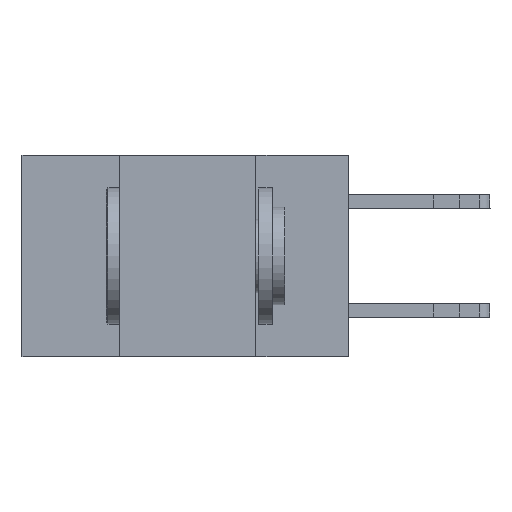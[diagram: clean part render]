
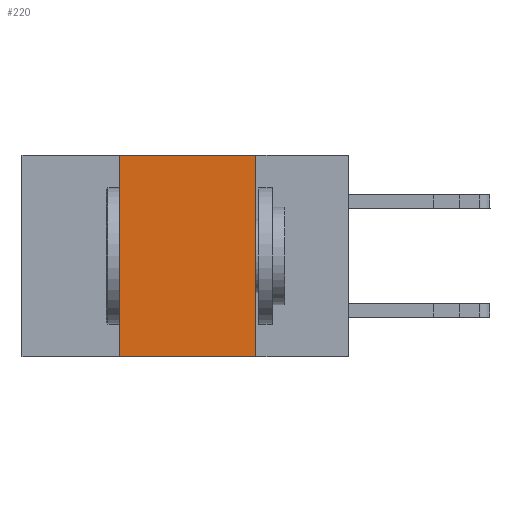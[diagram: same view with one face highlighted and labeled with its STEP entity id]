
A CAD part, left-side view. The second image highlights one B-rep face of the part: STEP entity #220.
In plain terms, the highlighted planar face has unit normal (-1, 0, 0).
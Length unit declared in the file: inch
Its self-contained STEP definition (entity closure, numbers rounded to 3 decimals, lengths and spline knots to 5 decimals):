
#20 = VECTOR ( 'NONE', #7049, 39.37008 ) ;
#220 = ADVANCED_FACE ( 'NONE', ( #6850 ), #9787, .F. ) ;
#585 = CARTESIAN_POINT ( 'NONE',  ( 0., 0.17, 0. ) ) ;
#595 = VECTOR ( 'NONE', #6662, 39.37008 ) ;
#762 = VERTEX_POINT ( 'NONE', #4689 ) ;
#771 = EDGE_CURVE ( 'NONE', #916, #762, #3615, .T. ) ;
#916 = VERTEX_POINT ( 'NONE', #2833 ) ;
#1364 = DIRECTION ( 'NONE',  ( 0., 0., -1. ) ) ;
#2590 = EDGE_CURVE ( 'NONE', #7582, #5184, #9550, .T. ) ;
#2833 = CARTESIAN_POINT ( 'NONE',  ( 0., 0.42, 0. ) ) ;
#3352 = ORIENTED_EDGE ( 'NONE', *, *, #8209, .F. ) ;
#3392 = VECTOR ( 'NONE', #8274, 39.37008 ) ;
#3615 = LINE ( 'NONE', #11863, #3392 ) ;
#3619 = EDGE_CURVE ( 'NONE', #7582, #916, #7566, .T. ) ;
#4126 = DIRECTION ( 'NONE',  ( 1., 0., 0. ) ) ;
#4689 = CARTESIAN_POINT ( 'NONE',  ( 0., 0.17, 0. ) ) ;
#4822 = CARTESIAN_POINT ( 'NONE',  ( 0., 0.42, -0.37 ) ) ;
#5128 = AXIS2_PLACEMENT_3D ( 'NONE', #5946, #4126, #1364 ) ;
#5137 = ORIENTED_EDGE ( 'NONE', *, *, #3619, .F. ) ;
#5160 = LINE ( 'NONE', #585, #20 ) ;
#5184 = VERTEX_POINT ( 'NONE', #9197 ) ;
#5752 = ORIENTED_EDGE ( 'NONE', *, *, #771, .F. ) ;
#5946 = CARTESIAN_POINT ( 'NONE',  ( 0., 0.6, 0. ) ) ;
#6662 = DIRECTION ( 'NONE',  ( 0., 0., 1. ) ) ;
#6850 = FACE_OUTER_BOUND ( 'NONE', #9932, .T. ) ;
#7049 = DIRECTION ( 'NONE',  ( 0., 0., -1. ) ) ;
#7566 = LINE ( 'NONE', #7737, #595 ) ;
#7582 = VERTEX_POINT ( 'NONE', #4822 ) ;
#7624 = VECTOR ( 'NONE', #7886, 39.37008 ) ;
#7655 = CARTESIAN_POINT ( 'NONE',  ( 0., 0.6, -0.37 ) ) ;
#7737 = CARTESIAN_POINT ( 'NONE',  ( 0., 0.42, 0. ) ) ;
#7886 = DIRECTION ( 'NONE',  ( 0., -1., 0. ) ) ;
#8209 = EDGE_CURVE ( 'NONE', #762, #5184, #5160, .T. ) ;
#8274 = DIRECTION ( 'NONE',  ( 0., -1., 0. ) ) ;
#8460 = ORIENTED_EDGE ( 'NONE', *, *, #2590, .T. ) ;
#9197 = CARTESIAN_POINT ( 'NONE',  ( 0., 0.17, -0.37 ) ) ;
#9550 = LINE ( 'NONE', #7655, #7624 ) ;
#9787 = PLANE ( 'NONE',  #5128 ) ;
#9932 = EDGE_LOOP ( 'NONE', ( #3352, #5752, #5137, #8460 ) ) ;
#11863 = CARTESIAN_POINT ( 'NONE',  ( 0., 0.6, 0. ) ) ;
